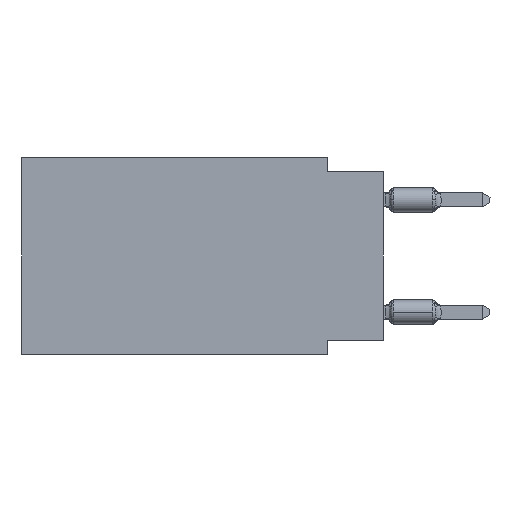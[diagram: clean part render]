
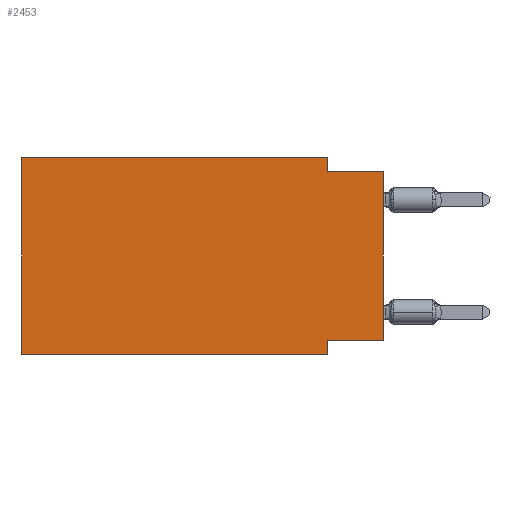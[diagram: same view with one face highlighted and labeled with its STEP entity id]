
A CAD part, left-side view. The second image highlights one B-rep face of the part: STEP entity #2453.
In plain terms, the highlighted planar face has unit normal (-1, 0, 0).
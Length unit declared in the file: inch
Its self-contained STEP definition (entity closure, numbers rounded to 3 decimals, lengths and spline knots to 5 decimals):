
#357 = LINE ( 'NONE', #1881, #5440 ) ;
#910 = CARTESIAN_POINT ( 'NONE',  ( 0., 0.1, 0. ) ) ;
#921 = DIRECTION ( 'NONE',  ( 0., -1., 0. ) ) ;
#1223 = CARTESIAN_POINT ( 'NONE',  ( 0., 0.645, -0.35 ) ) ;
#1881 = CARTESIAN_POINT ( 'NONE',  ( 0., 0., 0. ) ) ;
#2034 = CARTESIAN_POINT ( 'NONE',  ( 0., 0.1, -0.325 ) ) ;
#2453 = ADVANCED_FACE ( 'NONE', ( #10612 ), #3050, .F. ) ;
#2680 = VECTOR ( 'NONE', #10400, 39.37008 ) ;
#3050 = PLANE ( 'NONE',  #7580 ) ;
#4586 = EDGE_CURVE ( 'NONE', #11850, #9099, #6887, .T. ) ;
#5226 = VECTOR ( 'NONE', #921, 39.37008 ) ;
#5440 = VECTOR ( 'NONE', #18825, 39.37008 ) ;
#5582 = EDGE_CURVE ( 'NONE', #16474, #7499, #13752, .T. ) ;
#5693 = VERTEX_POINT ( 'NONE', #18516 ) ;
#5821 = EDGE_CURVE ( 'NONE', #11820, #12422, #13045, .T. ) ;
#5911 = EDGE_CURVE ( 'NONE', #5693, #11820, #11239, .T. ) ;
#5979 = ORIENTED_EDGE ( 'NONE', *, *, #17526, .F. ) ;
#6509 = VERTEX_POINT ( 'NONE', #15891 ) ;
#6887 = LINE ( 'NONE', #19196, #5226 ) ;
#7041 = ORIENTED_EDGE ( 'NONE', *, *, #4586, .F. ) ;
#7052 = CARTESIAN_POINT ( 'NONE',  ( 0., 0.645, 0. ) ) ;
#7303 = ORIENTED_EDGE ( 'NONE', *, *, #5911, .F. ) ;
#7499 = VERTEX_POINT ( 'NONE', #910 ) ;
#7580 = AXIS2_PLACEMENT_3D ( 'NONE', #16762, #8924, #12030 ) ;
#7776 = ORIENTED_EDGE ( 'NONE', *, *, #10614, .T. ) ;
#8227 = CARTESIAN_POINT ( 'NONE',  ( 0., 0.645, 0. ) ) ;
#8924 = DIRECTION ( 'NONE',  ( 1., 0., 0. ) ) ;
#8961 = CARTESIAN_POINT ( 'NONE',  ( 0., 0.1, -0.35 ) ) ;
#9030 = VECTOR ( 'NONE', #17682, 39.37008 ) ;
#9099 = VERTEX_POINT ( 'NONE', #11448 ) ;
#9177 = ORIENTED_EDGE ( 'NONE', *, *, #5821, .F. ) ;
#9323 = DIRECTION ( 'NONE',  ( 0., 0., -1. ) ) ;
#9915 = CARTESIAN_POINT ( 'NONE',  ( 0., 0.1, -0.35 ) ) ;
#10332 = VECTOR ( 'NONE', #19925, 39.37008 ) ;
#10400 = DIRECTION ( 'NONE',  ( 0., -1., 0. ) ) ;
#10612 = FACE_OUTER_BOUND ( 'NONE', #13702, .T. ) ;
#10614 = EDGE_CURVE ( 'NONE', #5693, #9099, #357, .T. ) ;
#10624 = ORIENTED_EDGE ( 'NONE', *, *, #19882, .F. ) ;
#10655 = VECTOR ( 'NONE', #9323, 39.37008 ) ;
#11239 = LINE ( 'NONE', #17393, #14499 ) ;
#11448 = CARTESIAN_POINT ( 'NONE',  ( 0., 0., -0.025 ) ) ;
#11820 = VERTEX_POINT ( 'NONE', #2034 ) ;
#11850 = VERTEX_POINT ( 'NONE', #13309 ) ;
#12030 = DIRECTION ( 'NONE',  ( 0., 0., -1. ) ) ;
#12422 = VERTEX_POINT ( 'NONE', #8961 ) ;
#12446 = LINE ( 'NONE', #12751, #10655 ) ;
#12751 = CARTESIAN_POINT ( 'NONE',  ( 0., 0.1, 0. ) ) ;
#12985 = EDGE_CURVE ( 'NONE', #6509, #12422, #18170, .T. ) ;
#13045 = LINE ( 'NONE', #9915, #9030 ) ;
#13309 = CARTESIAN_POINT ( 'NONE',  ( 0., 0.1, -0.025 ) ) ;
#13663 = CARTESIAN_POINT ( 'NONE',  ( 0., 0.645, 0. ) ) ;
#13702 = EDGE_LOOP ( 'NONE', ( #7776, #7041, #5979, #18696, #10624, #19869, #9177, #7303 ) ) ;
#13752 = LINE ( 'NONE', #13663, #10332 ) ;
#14463 = DIRECTION ( 'NONE',  ( 0., 1., 0. ) ) ;
#14499 = VECTOR ( 'NONE', #14463, 39.37008 ) ;
#14713 = LINE ( 'NONE', #7052, #19457 ) ;
#15891 = CARTESIAN_POINT ( 'NONE',  ( 0., 0.645, -0.35 ) ) ;
#16351 = DIRECTION ( 'NONE',  ( 0., 0., 1. ) ) ;
#16474 = VERTEX_POINT ( 'NONE', #8227 ) ;
#16762 = CARTESIAN_POINT ( 'NONE',  ( 0., 0.645, 0. ) ) ;
#17393 = CARTESIAN_POINT ( 'NONE',  ( 0., 0., -0.325 ) ) ;
#17526 = EDGE_CURVE ( 'NONE', #7499, #11850, #12446, .T. ) ;
#17682 = DIRECTION ( 'NONE',  ( 0., 0., -1. ) ) ;
#18170 = LINE ( 'NONE', #1223, #2680 ) ;
#18516 = CARTESIAN_POINT ( 'NONE',  ( 0., 0., -0.325 ) ) ;
#18696 = ORIENTED_EDGE ( 'NONE', *, *, #5582, .F. ) ;
#18825 = DIRECTION ( 'NONE',  ( 0., 0., 1. ) ) ;
#19196 = CARTESIAN_POINT ( 'NONE',  ( 0., 0., -0.025 ) ) ;
#19457 = VECTOR ( 'NONE', #16351, 39.37008 ) ;
#19869 = ORIENTED_EDGE ( 'NONE', *, *, #12985, .T. ) ;
#19882 = EDGE_CURVE ( 'NONE', #6509, #16474, #14713, .T. ) ;
#19925 = DIRECTION ( 'NONE',  ( 0., -1., 0. ) ) ;
